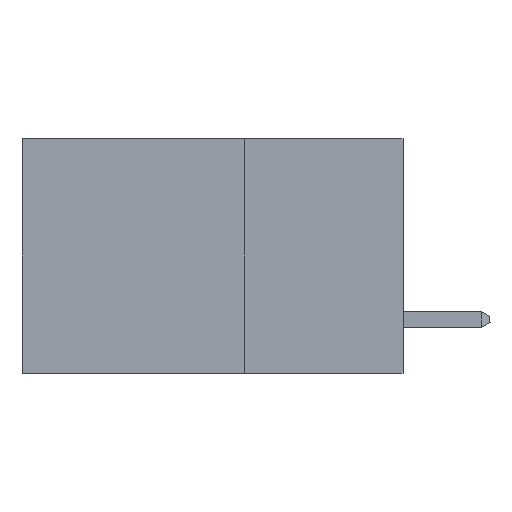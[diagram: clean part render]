
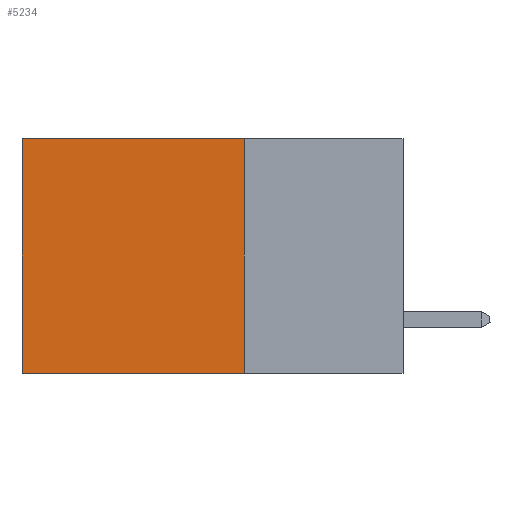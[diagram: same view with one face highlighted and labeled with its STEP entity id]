
A CAD part, left-side view. The second image highlights one B-rep face of the part: STEP entity #5234.
In plain terms, the highlighted planar face has unit normal (-1, 0, 0).
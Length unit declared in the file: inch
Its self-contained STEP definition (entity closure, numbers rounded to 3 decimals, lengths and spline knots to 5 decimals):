
#800 = DIRECTION ( 'NONE',  ( 1., 0., 0. ) ) ;
#1012 = AXIS2_PLACEMENT_3D ( 'NONE', #30891, #800, #21981 ) ;
#1123 = FACE_OUTER_BOUND ( 'NONE', #21144, .T. ) ;
#1145 = LINE ( 'NONE', #10534, #32310 ) ;
#1189 = LINE ( 'NONE', #30678, #23429 ) ;
#1419 = ORIENTED_EDGE ( 'NONE', *, *, #14140, .F. ) ;
#5234 = ADVANCED_FACE ( 'NONE', ( #1123 ), #36894, .F. ) ;
#6805 = ORIENTED_EDGE ( 'NONE', *, *, #30906, .T. ) ;
#7346 = VERTEX_POINT ( 'NONE', #32672 ) ;
#8091 = LINE ( 'NONE', #24500, #23067 ) ;
#9849 = CARTESIAN_POINT ( 'NONE',  ( 0.2875, 0.6, -0.37 ) ) ;
#10534 = CARTESIAN_POINT ( 'NONE',  ( 0.2875, 0.6, 0. ) ) ;
#10715 = VERTEX_POINT ( 'NONE', #36548 ) ;
#11655 = CARTESIAN_POINT ( 'NONE',  ( 0.2875, 0.25, -0.37 ) ) ;
#12763 = DIRECTION ( 'NONE',  ( 0., 0., -1. ) ) ;
#14140 = EDGE_CURVE ( 'NONE', #32040, #30994, #32254, .T. ) ;
#14486 = VECTOR ( 'NONE', #30999, 39.37008 ) ;
#20733 = ORIENTED_EDGE ( 'NONE', *, *, #36899, .F. ) ;
#21144 = EDGE_LOOP ( 'NONE', ( #31946, #1419, #20733, #6805 ) ) ;
#21981 = DIRECTION ( 'NONE',  ( 0., 0., -1. ) ) ;
#23067 = VECTOR ( 'NONE', #27554, 39.37008 ) ;
#23429 = VECTOR ( 'NONE', #12763, 39.37008 ) ;
#24500 = CARTESIAN_POINT ( 'NONE',  ( 0.2875, 0.25, 0. ) ) ;
#24950 = CARTESIAN_POINT ( 'NONE',  ( 0.2875, 0.25, -0.37 ) ) ;
#27554 = DIRECTION ( 'NONE',  ( 0., 1., 0. ) ) ;
#30678 = CARTESIAN_POINT ( 'NONE',  ( 0.2875, 0.25, 0. ) ) ;
#30891 = CARTESIAN_POINT ( 'NONE',  ( 0.2875, 0.25, 0. ) ) ;
#30906 = EDGE_CURVE ( 'NONE', #7346, #10715, #8091, .T. ) ;
#30994 = VERTEX_POINT ( 'NONE', #9849 ) ;
#30999 = DIRECTION ( 'NONE',  ( 0., 1., 0. ) ) ;
#31946 = ORIENTED_EDGE ( 'NONE', *, *, #32752, .T. ) ;
#32040 = VERTEX_POINT ( 'NONE', #11655 ) ;
#32254 = LINE ( 'NONE', #24950, #14486 ) ;
#32310 = VECTOR ( 'NONE', #37478, 39.37008 ) ;
#32672 = CARTESIAN_POINT ( 'NONE',  ( 0.2875, 0.25, 0. ) ) ;
#32752 = EDGE_CURVE ( 'NONE', #10715, #30994, #1145, .T. ) ;
#36548 = CARTESIAN_POINT ( 'NONE',  ( 0.2875, 0.6, 0. ) ) ;
#36894 = PLANE ( 'NONE',  #1012 ) ;
#36899 = EDGE_CURVE ( 'NONE', #7346, #32040, #1189, .T. ) ;
#37478 = DIRECTION ( 'NONE',  ( 0., 0., -1. ) ) ;
